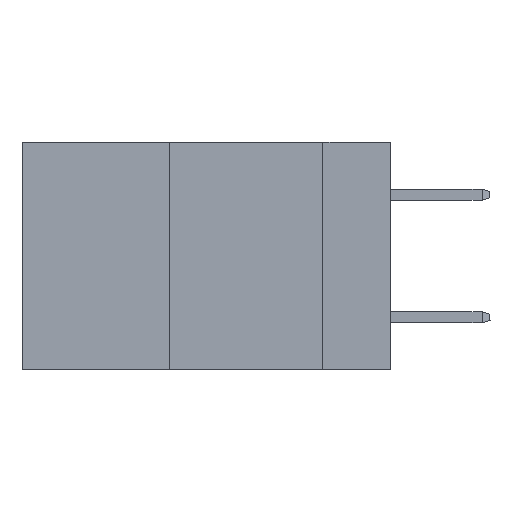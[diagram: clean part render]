
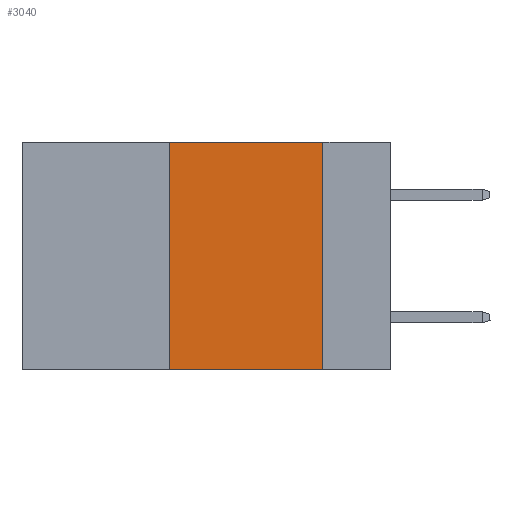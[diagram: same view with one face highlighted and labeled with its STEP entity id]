
A CAD part, left-side view. The second image highlights one B-rep face of the part: STEP entity #3040.
In plain terms, the highlighted planar face has unit normal (-1, 0, 0).
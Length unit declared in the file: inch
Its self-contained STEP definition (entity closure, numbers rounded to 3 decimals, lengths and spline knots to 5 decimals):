
#522 = DIRECTION ( 'NONE',  ( 0., -1., 0. ) ) ;
#631 = EDGE_CURVE ( 'NONE', #16454, #4345, #5775, .T. ) ;
#1211 = CARTESIAN_POINT ( 'NONE',  ( 0., 0.36, -0.37 ) ) ;
#1249 = VECTOR ( 'NONE', #522, 39.37008 ) ;
#1666 = CARTESIAN_POINT ( 'NONE',  ( 0., 0.36, 0. ) ) ;
#1848 = DIRECTION ( 'NONE',  ( 1., 0., 0. ) ) ;
#2779 = DIRECTION ( 'NONE',  ( 0., 0., -1. ) ) ;
#3040 = ADVANCED_FACE ( 'NONE', ( #3798 ), #19036, .F. ) ;
#3134 = VECTOR ( 'NONE', #11812, 39.37008 ) ;
#3798 = FACE_OUTER_BOUND ( 'NONE', #12037, .T. ) ;
#4345 = VERTEX_POINT ( 'NONE', #6732 ) ;
#5775 = LINE ( 'NONE', #7433, #3134 ) ;
#6732 = CARTESIAN_POINT ( 'NONE',  ( 0., 0.11, 0. ) ) ;
#7152 = CARTESIAN_POINT ( 'NONE',  ( 0., 0.11, 0. ) ) ;
#7158 = ORIENTED_EDGE ( 'NONE', *, *, #7649, .F. ) ;
#7433 = CARTESIAN_POINT ( 'NONE',  ( 0., 0.6, 0. ) ) ;
#7649 = EDGE_CURVE ( 'NONE', #4345, #10702, #16724, .T. ) ;
#8089 = DIRECTION ( 'NONE',  ( 0., 0., -1. ) ) ;
#8181 = EDGE_CURVE ( 'NONE', #8981, #16454, #15136, .T. ) ;
#8981 = VERTEX_POINT ( 'NONE', #1211 ) ;
#10702 = VERTEX_POINT ( 'NONE', #10966 ) ;
#10966 = CARTESIAN_POINT ( 'NONE',  ( 0., 0.11, -0.37 ) ) ;
#10982 = AXIS2_PLACEMENT_3D ( 'NONE', #11129, #1848, #8089 ) ;
#11129 = CARTESIAN_POINT ( 'NONE',  ( 0., 0.6, 0. ) ) ;
#11812 = DIRECTION ( 'NONE',  ( 0., -1., 0. ) ) ;
#11881 = CARTESIAN_POINT ( 'NONE',  ( 0., 0.6, -0.37 ) ) ;
#12037 = EDGE_LOOP ( 'NONE', ( #7158, #20058, #13887, #19602 ) ) ;
#12114 = VECTOR ( 'NONE', #18479, 39.37008 ) ;
#13442 = LINE ( 'NONE', #11881, #1249 ) ;
#13887 = ORIENTED_EDGE ( 'NONE', *, *, #8181, .F. ) ;
#15136 = LINE ( 'NONE', #16483, #12114 ) ;
#16454 = VERTEX_POINT ( 'NONE', #1666 ) ;
#16483 = CARTESIAN_POINT ( 'NONE',  ( 0., 0.36, 0. ) ) ;
#16724 = LINE ( 'NONE', #7152, #17788 ) ;
#17788 = VECTOR ( 'NONE', #2779, 39.37008 ) ;
#18479 = DIRECTION ( 'NONE',  ( 0., 0., 1. ) ) ;
#19036 = PLANE ( 'NONE',  #10982 ) ;
#19593 = EDGE_CURVE ( 'NONE', #8981, #10702, #13442, .T. ) ;
#19602 = ORIENTED_EDGE ( 'NONE', *, *, #19593, .T. ) ;
#20058 = ORIENTED_EDGE ( 'NONE', *, *, #631, .F. ) ;
